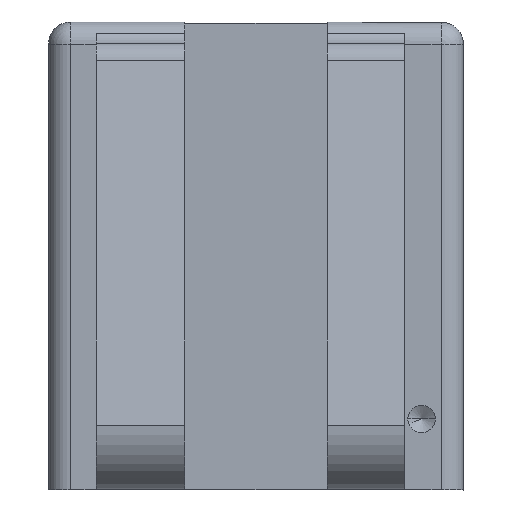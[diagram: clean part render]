
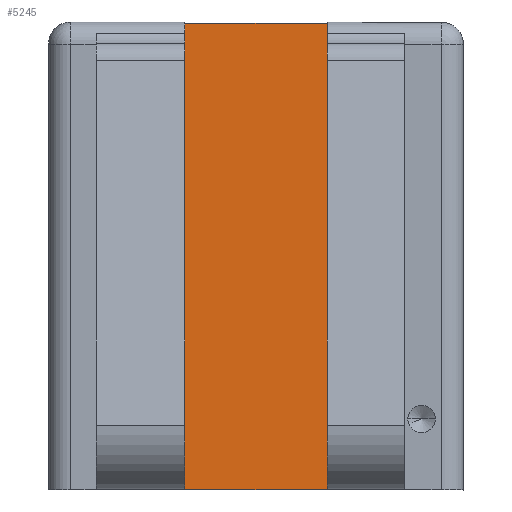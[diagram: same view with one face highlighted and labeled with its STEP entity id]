
A CAD part, front view. The second image highlights one B-rep face of the part: STEP entity #5245.
In plain terms, the highlighted planar face has unit normal (0, -1, 0).
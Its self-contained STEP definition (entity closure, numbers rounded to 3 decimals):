
#29 = LINE ( 'NONE', #3205, #5899 ) ;
#536 = EDGE_LOOP ( 'NONE', ( #3312, #2384, #6712, #3195 ) ) ;
#580 = CARTESIAN_POINT ( 'NONE',  ( 5.69, -45.041, 238.244 ) ) ;
#947 = FACE_OUTER_BOUND ( 'NONE', #536, .T. ) ;
#1104 = VECTOR ( 'NONE', #3777, 1000. ) ;
#1212 = VERTEX_POINT ( 'NONE', #3046 ) ;
#1505 = EDGE_CURVE ( 'NONE', #1212, #1619, #3753, .T. ) ;
#1609 = PLANE ( 'NONE',  #8367 ) ;
#1619 = VERTEX_POINT ( 'NONE', #5585 ) ;
#1640 = DIRECTION ( 'NONE',  ( 1., 0., 0. ) ) ;
#2384 = ORIENTED_EDGE ( 'NONE', *, *, #1505, .T. ) ;
#2708 = LINE ( 'NONE', #3854, #8738 ) ;
#3046 = CARTESIAN_POINT ( 'NONE',  ( 5.69, -45.041, 196.506 ) ) ;
#3195 = ORIENTED_EDGE ( 'NONE', *, *, #9296, .F. ) ;
#3203 = CARTESIAN_POINT ( 'NONE',  ( 5.69, -45.041, 196.506 ) ) ;
#3205 = CARTESIAN_POINT ( 'NONE',  ( -4.526, -45.041, 238.244 ) ) ;
#3312 = ORIENTED_EDGE ( 'NONE', *, *, #5125, .T. ) ;
#3493 = VERTEX_POINT ( 'NONE', #8311 ) ;
#3597 = LINE ( 'NONE', #3203, #9352 ) ;
#3753 = LINE ( 'NONE', #6105, #1104 ) ;
#3777 = DIRECTION ( 'NONE',  ( 1., 0., 0. ) ) ;
#3854 = CARTESIAN_POINT ( 'NONE',  ( 18.39, -45.041, 196.506 ) ) ;
#4027 = DIRECTION ( 'NONE',  ( 0., 0., -1. ) ) ;
#5125 = EDGE_CURVE ( 'NONE', #8270, #1212, #3597, .T. ) ;
#5245 = ADVANCED_FACE ( 'NONE', ( #947 ), #1609, .T. ) ;
#5585 = CARTESIAN_POINT ( 'NONE',  ( 18.39, -45.041, 196.506 ) ) ;
#5693 = EDGE_CURVE ( 'NONE', #3493, #1619, #2708, .T. ) ;
#5899 = VECTOR ( 'NONE', #8709, 1000. ) ;
#6105 = CARTESIAN_POINT ( 'NONE',  ( -38.566, -45.041, 196.506 ) ) ;
#6409 = DIRECTION ( 'NONE',  ( 0., -1., 0. ) ) ;
#6712 = ORIENTED_EDGE ( 'NONE', *, *, #5693, .F. ) ;
#8270 = VERTEX_POINT ( 'NONE', #580 ) ;
#8311 = CARTESIAN_POINT ( 'NONE',  ( 18.39, -45.041, 238.244 ) ) ;
#8367 = AXIS2_PLACEMENT_3D ( 'NONE', #9502, #6409, #1640 ) ;
#8547 = DIRECTION ( 'NONE',  ( 0., 0., -1. ) ) ;
#8709 = DIRECTION ( 'NONE',  ( 1., 0., 0. ) ) ;
#8738 = VECTOR ( 'NONE', #8547, 1000. ) ;
#9296 = EDGE_CURVE ( 'NONE', #8270, #3493, #29, .T. ) ;
#9352 = VECTOR ( 'NONE', #4027, 1000. ) ;
#9502 = CARTESIAN_POINT ( 'NONE',  ( -38.566, -45.041, 196.506 ) ) ;
